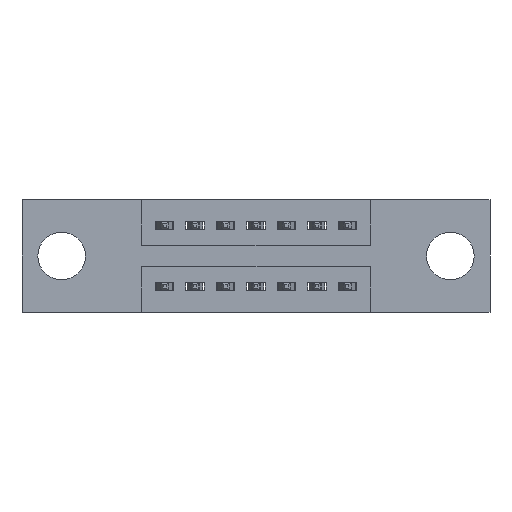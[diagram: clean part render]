
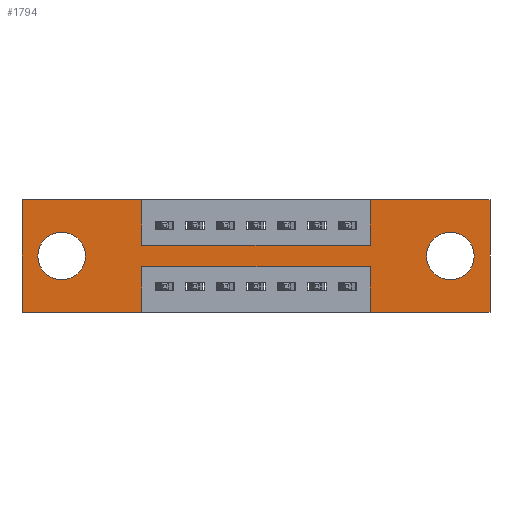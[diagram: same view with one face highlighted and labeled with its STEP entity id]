
A CAD part, front view. The second image highlights one B-rep face of the part: STEP entity #1794.
In plain terms, the highlighted planar face has unit normal (0, -1, 0).
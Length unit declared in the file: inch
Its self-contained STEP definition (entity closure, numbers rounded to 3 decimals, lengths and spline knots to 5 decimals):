
#99 = VECTOR ( 'NONE', #9262, 39.37008 ) ;
#176 = CIRCLE ( 'NONE', #10151, 0.078 ) ;
#260 = CARTESIAN_POINT ( 'NONE',  ( 1.1425, 0., -0.37 ) ) ;
#470 = CARTESIAN_POINT ( 'NONE',  ( 0., 0., 0. ) ) ;
#525 = VECTOR ( 'NONE', #4700, 39.37008 ) ;
#560 = LINE ( 'NONE', #8916, #4042 ) ;
#627 = CARTESIAN_POINT ( 'NONE',  ( 1.1425, 0., 0. ) ) ;
#632 = VERTEX_POINT ( 'NONE', #7097 ) ;
#652 = CARTESIAN_POINT ( 'NONE',  ( 0.3925, 0., 0. ) ) ;
#688 = CARTESIAN_POINT ( 'NONE',  ( 0.3925, 0., -0.37 ) ) ;
#772 = EDGE_CURVE ( 'NONE', #5098, #632, #1483, .T. ) ;
#787 = EDGE_CURVE ( 'NONE', #2264, #9590, #2910, .T. ) ;
#794 = ORIENTED_EDGE ( 'NONE', *, *, #787, .F. ) ;
#848 = CARTESIAN_POINT ( 'NONE',  ( 0.13, 0., -0.263 ) ) ;
#926 = CARTESIAN_POINT ( 'NONE',  ( 0.3925, 0., -0.37 ) ) ;
#973 = DIRECTION ( 'NONE',  ( 0., 1., 0. ) ) ;
#984 = CARTESIAN_POINT ( 'NONE',  ( 1.535, 0., -0.37 ) ) ;
#1186 = EDGE_CURVE ( 'NONE', #3671, #4750, #4225, .T. ) ;
#1197 = CARTESIAN_POINT ( 'NONE',  ( 1.535, 0., 0. ) ) ;
#1401 = CARTESIAN_POINT ( 'NONE',  ( 1.535, 0., 0. ) ) ;
#1483 = CIRCLE ( 'NONE', #4259, 0.078 ) ;
#1529 = DIRECTION ( 'NONE',  ( 1., 0., 0. ) ) ;
#1609 = CARTESIAN_POINT ( 'NONE',  ( 0.13, 0., -0.185 ) ) ;
#1794 = ADVANCED_FACE ( 'NONE', ( #6238, #1965, #7744 ), #8539, .T. ) ;
#1828 = AXIS2_PLACEMENT_3D ( 'NONE', #9284, #4307, #9187 ) ;
#1965 = FACE_BOUND ( 'NONE', #5969, .T. ) ;
#1995 = VERTEX_POINT ( 'NONE', #3322 ) ;
#2001 = CIRCLE ( 'NONE', #1828, 0.078 ) ;
#2095 = VERTEX_POINT ( 'NONE', #5186 ) ;
#2221 = CARTESIAN_POINT ( 'NONE',  ( 0., 0., 0. ) ) ;
#2264 = VERTEX_POINT ( 'NONE', #1401 ) ;
#2269 = EDGE_CURVE ( 'NONE', #3099, #2264, #6324, .T. ) ;
#2272 = CARTESIAN_POINT ( 'NONE',  ( 1.1425, 0., -0.37 ) ) ;
#2288 = LINE ( 'NONE', #627, #7364 ) ;
#2395 = CARTESIAN_POINT ( 'NONE',  ( 0.13, 0., -0.107 ) ) ;
#2523 = AXIS2_PLACEMENT_3D ( 'NONE', #10169, #9510, #2767 ) ;
#2704 = CARTESIAN_POINT ( 'NONE',  ( 1.405, 0., -0.185 ) ) ;
#2726 = DIRECTION ( 'NONE',  ( 0., 0., -1. ) ) ;
#2767 = DIRECTION ( 'NONE',  ( 0., 0., -1. ) ) ;
#2858 = DIRECTION ( 'NONE',  ( 0., 0., -1. ) ) ;
#2910 = LINE ( 'NONE', #1197, #3026 ) ;
#2960 = EDGE_CURVE ( 'NONE', #632, #5098, #176, .T. ) ;
#3026 = VECTOR ( 'NONE', #2858, 39.37008 ) ;
#3083 = DIRECTION ( 'NONE',  ( 0., 0., 1. ) ) ;
#3099 = VERTEX_POINT ( 'NONE', #7285 ) ;
#3284 = ORIENTED_EDGE ( 'NONE', *, *, #2269, .F. ) ;
#3311 = DIRECTION ( 'NONE',  ( 0., 1., 0. ) ) ;
#3322 = CARTESIAN_POINT ( 'NONE',  ( 1.1425, 0., -0.15 ) ) ;
#3334 = VECTOR ( 'NONE', #2726, 39.37008 ) ;
#3348 = CARTESIAN_POINT ( 'NONE',  ( 0., 0., -0.37 ) ) ;
#3443 = CARTESIAN_POINT ( 'NONE',  ( 1.1425, 0., -0.22 ) ) ;
#3584 = LINE ( 'NONE', #7600, #3334 ) ;
#3592 = ORIENTED_EDGE ( 'NONE', *, *, #8386, .F. ) ;
#3671 = VERTEX_POINT ( 'NONE', #688 ) ;
#3754 = DIRECTION ( 'NONE',  ( 0., 0., 1. ) ) ;
#3760 = EDGE_LOOP ( 'NONE', ( #4127, #8965, #7820, #6188, #794, #3284, #5849, #7107, #5940, #3994, #3592, #3941 ) ) ;
#3941 = ORIENTED_EDGE ( 'NONE', *, *, #1186, .F. ) ;
#3994 = ORIENTED_EDGE ( 'NONE', *, *, #4192, .F. ) ;
#4042 = VECTOR ( 'NONE', #1529, 39.37008 ) ;
#4127 = ORIENTED_EDGE ( 'NONE', *, *, #9972, .F. ) ;
#4135 = EDGE_CURVE ( 'NONE', #2095, #1995, #10588, .T. ) ;
#4192 = EDGE_CURVE ( 'NONE', #7445, #6203, #560, .T. ) ;
#4225 = LINE ( 'NONE', #5180, #99 ) ;
#4259 = AXIS2_PLACEMENT_3D ( 'NONE', #2704, #8577, #5259 ) ;
#4307 = DIRECTION ( 'NONE',  ( 0., 1., 0. ) ) ;
#4502 = EDGE_CURVE ( 'NONE', #7357, #7336, #5698, .T. ) ;
#4599 = CARTESIAN_POINT ( 'NONE',  ( 0.3925, 0., -0.22 ) ) ;
#4700 = DIRECTION ( 'NONE',  ( 1., 0., 0. ) ) ;
#4750 = VERTEX_POINT ( 'NONE', #3348 ) ;
#4865 = DIRECTION ( 'NONE',  ( -1., 0., 0. ) ) ;
#4895 = EDGE_CURVE ( 'NONE', #6203, #2095, #3584, .T. ) ;
#5039 = CARTESIAN_POINT ( 'NONE',  ( 1.405, 0., -0.185 ) ) ;
#5098 = VERTEX_POINT ( 'NONE', #7058 ) ;
#5180 = CARTESIAN_POINT ( 'NONE',  ( 0., 0., -0.37 ) ) ;
#5186 = CARTESIAN_POINT ( 'NONE',  ( 0.3925, 0., -0.15 ) ) ;
#5222 = CARTESIAN_POINT ( 'NONE',  ( 0., 0., -0.37 ) ) ;
#5259 = DIRECTION ( 'NONE',  ( 0., 0., -1. ) ) ;
#5430 = EDGE_LOOP ( 'NONE', ( #6173, #7799 ) ) ;
#5451 = VERTEX_POINT ( 'NONE', #848 ) ;
#5652 = DIRECTION ( 'NONE',  ( 1., 0., 0. ) ) ;
#5698 = LINE ( 'NONE', #2272, #6792 ) ;
#5835 = VECTOR ( 'NONE', #7635, 39.37008 ) ;
#5849 = ORIENTED_EDGE ( 'NONE', *, *, #10158, .F. ) ;
#5940 = ORIENTED_EDGE ( 'NONE', *, *, #4895, .F. ) ;
#5969 = EDGE_LOOP ( 'NONE', ( #7134, #6273 ) ) ;
#6082 = VECTOR ( 'NONE', #5652, 39.37008 ) ;
#6173 = ORIENTED_EDGE ( 'NONE', *, *, #772, .T. ) ;
#6188 = ORIENTED_EDGE ( 'NONE', *, *, #10034, .F. ) ;
#6203 = VERTEX_POINT ( 'NONE', #652 ) ;
#6238 = FACE_BOUND ( 'NONE', #5430, .T. ) ;
#6273 = ORIENTED_EDGE ( 'NONE', *, *, #9987, .T. ) ;
#6324 = LINE ( 'NONE', #2221, #525 ) ;
#6551 = CARTESIAN_POINT ( 'NONE',  ( 0.3925, 0., -0.22 ) ) ;
#6566 = DIRECTION ( 'NONE',  ( 0., 0., -1. ) ) ;
#6685 = VECTOR ( 'NONE', #3754, 39.37008 ) ;
#6792 = VECTOR ( 'NONE', #8148, 39.37008 ) ;
#7058 = CARTESIAN_POINT ( 'NONE',  ( 1.405, 0., -0.107 ) ) ;
#7097 = CARTESIAN_POINT ( 'NONE',  ( 1.405, 0., -0.263 ) ) ;
#7107 = ORIENTED_EDGE ( 'NONE', *, *, #4135, .F. ) ;
#7134 = ORIENTED_EDGE ( 'NONE', *, *, #8576, .T. ) ;
#7285 = CARTESIAN_POINT ( 'NONE',  ( 1.1425, 0., 0. ) ) ;
#7336 = VERTEX_POINT ( 'NONE', #3443 ) ;
#7357 = VERTEX_POINT ( 'NONE', #260 ) ;
#7364 = VECTOR ( 'NONE', #3083, 39.37008 ) ;
#7402 = DIRECTION ( 'NONE',  ( 0., 0., 1. ) ) ;
#7445 = VERTEX_POINT ( 'NONE', #8722 ) ;
#7531 = AXIS2_PLACEMENT_3D ( 'NONE', #1609, #973, #7402 ) ;
#7600 = CARTESIAN_POINT ( 'NONE',  ( 0.3925, 0., 0. ) ) ;
#7635 = DIRECTION ( 'NONE',  ( -1., 0., 0. ) ) ;
#7744 = FACE_OUTER_BOUND ( 'NONE', #3760, .T. ) ;
#7799 = ORIENTED_EDGE ( 'NONE', *, *, #2960, .T. ) ;
#7820 = ORIENTED_EDGE ( 'NONE', *, *, #4502, .F. ) ;
#7880 = VERTEX_POINT ( 'NONE', #4599 ) ;
#8148 = DIRECTION ( 'NONE',  ( 0., 0., 1. ) ) ;
#8386 = EDGE_CURVE ( 'NONE', #4750, #7445, #10376, .T. ) ;
#8396 = DIRECTION ( 'NONE',  ( 0., 0., -1. ) ) ;
#8524 = VECTOR ( 'NONE', #4865, 39.37008 ) ;
#8539 = PLANE ( 'NONE',  #2523 ) ;
#8576 = EDGE_CURVE ( 'NONE', #9079, #5451, #2001, .T. ) ;
#8577 = DIRECTION ( 'NONE',  ( 0., 1., 0. ) ) ;
#8722 = CARTESIAN_POINT ( 'NONE',  ( 0., 0., 0. ) ) ;
#8848 = LINE ( 'NONE', #6551, #8524 ) ;
#8891 = VECTOR ( 'NONE', #8396, 39.37008 ) ;
#8916 = CARTESIAN_POINT ( 'NONE',  ( 0., 0., 0. ) ) ;
#8965 = ORIENTED_EDGE ( 'NONE', *, *, #9486, .F. ) ;
#9079 = VERTEX_POINT ( 'NONE', #2395 ) ;
#9102 = LINE ( 'NONE', #926, #8891 ) ;
#9187 = DIRECTION ( 'NONE',  ( 0., 0., 1. ) ) ;
#9262 = DIRECTION ( 'NONE',  ( -1., 0., 0. ) ) ;
#9284 = CARTESIAN_POINT ( 'NONE',  ( 0.13, 0., -0.185 ) ) ;
#9348 = LINE ( 'NONE', #5222, #5835 ) ;
#9486 = EDGE_CURVE ( 'NONE', #7336, #7880, #8848, .T. ) ;
#9510 = DIRECTION ( 'NONE',  ( 0., -1., 0. ) ) ;
#9590 = VERTEX_POINT ( 'NONE', #984 ) ;
#9713 = CARTESIAN_POINT ( 'NONE',  ( 0.3925, 0., -0.15 ) ) ;
#9750 = CIRCLE ( 'NONE', #7531, 0.078 ) ;
#9972 = EDGE_CURVE ( 'NONE', #7880, #3671, #9102, .T. ) ;
#9987 = EDGE_CURVE ( 'NONE', #5451, #9079, #9750, .T. ) ;
#10034 = EDGE_CURVE ( 'NONE', #9590, #7357, #9348, .T. ) ;
#10151 = AXIS2_PLACEMENT_3D ( 'NONE', #5039, #3311, #6566 ) ;
#10158 = EDGE_CURVE ( 'NONE', #1995, #3099, #2288, .T. ) ;
#10169 = CARTESIAN_POINT ( 'NONE',  ( 0., 0., -0.37 ) ) ;
#10376 = LINE ( 'NONE', #470, #6685 ) ;
#10588 = LINE ( 'NONE', #9713, #6082 ) ;
